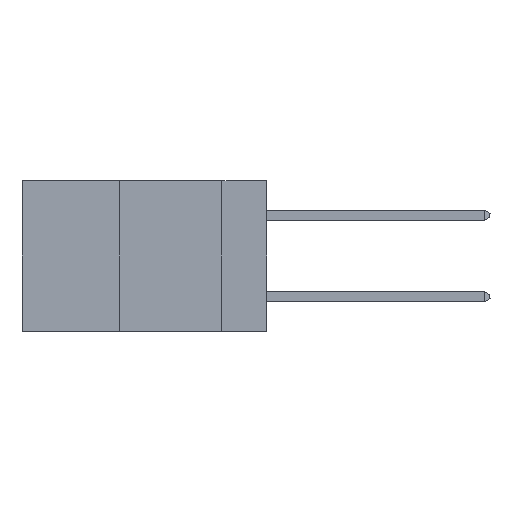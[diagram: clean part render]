
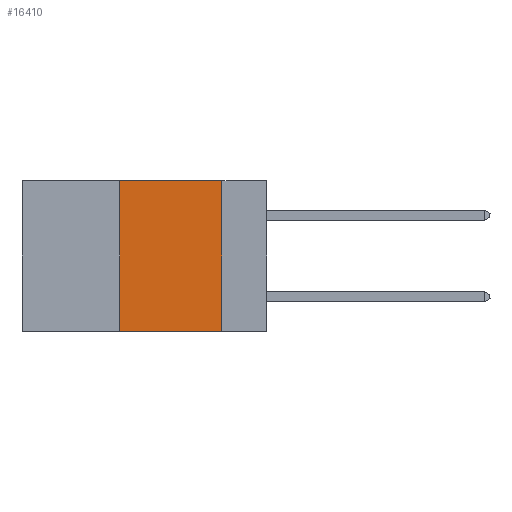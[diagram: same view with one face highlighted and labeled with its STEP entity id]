
A CAD part, left-side view. The second image highlights one B-rep face of the part: STEP entity #16410.
In plain terms, the highlighted planar face has unit normal (-1, 0, 0).
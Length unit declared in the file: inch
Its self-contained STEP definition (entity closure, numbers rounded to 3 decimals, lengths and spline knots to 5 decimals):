
#866 = VECTOR ( 'NONE', #39178, 39.37008 ) ;
#1322 = DIRECTION ( 'NONE',  ( 0., 0., -1. ) ) ;
#2471 = VERTEX_POINT ( 'NONE', #32526 ) ;
#2890 = CARTESIAN_POINT ( 'NONE',  ( 0., 0.11, 0. ) ) ;
#4258 = VECTOR ( 'NONE', #9419, 39.37008 ) ;
#4941 = DIRECTION ( 'NONE',  ( 1., 0., 0. ) ) ;
#6723 = EDGE_LOOP ( 'NONE', ( #29935, #12372, #33304, #23836 ) ) ;
#7455 = CARTESIAN_POINT ( 'NONE',  ( 0., 0.6, -0.37 ) ) ;
#8002 = EDGE_CURVE ( 'NONE', #12739, #2471, #28613, .T. ) ;
#9419 = DIRECTION ( 'NONE',  ( 0., 0., -1. ) ) ;
#10722 = DIRECTION ( 'NONE',  ( 0., -1., 0. ) ) ;
#12372 = ORIENTED_EDGE ( 'NONE', *, *, #22704, .F. ) ;
#12739 = VERTEX_POINT ( 'NONE', #35120 ) ;
#16181 = LINE ( 'NONE', #38838, #35930 ) ;
#16410 = ADVANCED_FACE ( 'NONE', ( #22412 ), #23993, .F. ) ;
#17148 = CARTESIAN_POINT ( 'NONE',  ( 0., 0.11, 0. ) ) ;
#17511 = CARTESIAN_POINT ( 'NONE',  ( 0., 0.6, 0. ) ) ;
#18982 = EDGE_CURVE ( 'NONE', #12739, #31299, #16181, .T. ) ;
#19804 = EDGE_CURVE ( 'NONE', #34051, #2471, #35850, .T. ) ;
#22412 = FACE_OUTER_BOUND ( 'NONE', #6723, .T. ) ;
#22704 = EDGE_CURVE ( 'NONE', #31299, #34051, #36579, .T. ) ;
#23836 = ORIENTED_EDGE ( 'NONE', *, *, #8002, .T. ) ;
#23993 = PLANE ( 'NONE',  #36138 ) ;
#28613 = LINE ( 'NONE', #7455, #866 ) ;
#28953 = CARTESIAN_POINT ( 'NONE',  ( 0., 0.6, 0. ) ) ;
#29935 = ORIENTED_EDGE ( 'NONE', *, *, #19804, .F. ) ;
#31299 = VERTEX_POINT ( 'NONE', #33685 ) ;
#32526 = CARTESIAN_POINT ( 'NONE',  ( 0., 0.11, -0.37 ) ) ;
#33304 = ORIENTED_EDGE ( 'NONE', *, *, #18982, .F. ) ;
#33685 = CARTESIAN_POINT ( 'NONE',  ( 0., 0.36, 0. ) ) ;
#34051 = VERTEX_POINT ( 'NONE', #2890 ) ;
#35120 = CARTESIAN_POINT ( 'NONE',  ( 0., 0.36, -0.37 ) ) ;
#35850 = LINE ( 'NONE', #17148, #4258 ) ;
#35930 = VECTOR ( 'NONE', #38573, 39.37008 ) ;
#36138 = AXIS2_PLACEMENT_3D ( 'NONE', #17511, #4941, #1322 ) ;
#36579 = LINE ( 'NONE', #28953, #37554 ) ;
#37554 = VECTOR ( 'NONE', #10722, 39.37008 ) ;
#38573 = DIRECTION ( 'NONE',  ( 0., 0., 1. ) ) ;
#38838 = CARTESIAN_POINT ( 'NONE',  ( 0., 0.36, 0. ) ) ;
#39178 = DIRECTION ( 'NONE',  ( 0., -1., 0. ) ) ;
